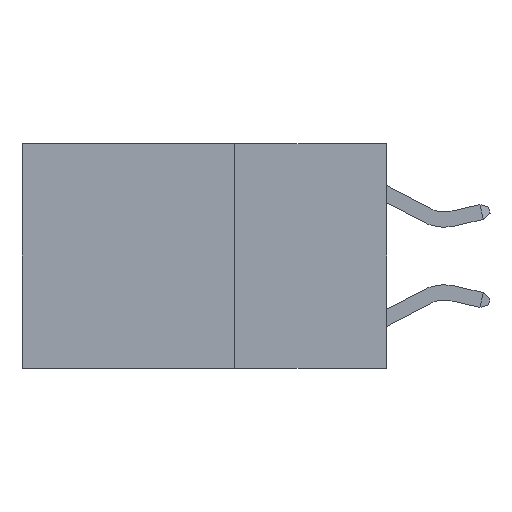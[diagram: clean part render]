
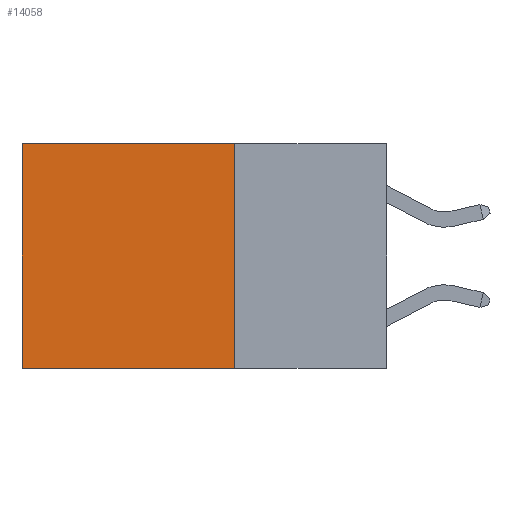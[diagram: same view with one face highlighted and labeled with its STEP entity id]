
A CAD part, left-side view. The second image highlights one B-rep face of the part: STEP entity #14058.
In plain terms, the highlighted planar face has unit normal (-1, 0, 0).
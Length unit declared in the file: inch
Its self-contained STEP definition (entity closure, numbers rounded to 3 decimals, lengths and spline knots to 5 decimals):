
#892 = EDGE_CURVE ( 'NONE', #7675, #2866, #4655, .T. ) ;
#1276 = AXIS2_PLACEMENT_3D ( 'NONE', #11040, #17095, #6116 ) ;
#1988 = EDGE_CURVE ( 'NONE', #10355, #12575, #14997, .T. ) ;
#2866 = VERTEX_POINT ( 'NONE', #5969 ) ;
#3152 = CARTESIAN_POINT ( 'NONE',  ( 0.2625, 0.25, -0.37 ) ) ;
#3820 = VECTOR ( 'NONE', #10582, 39.37008 ) ;
#3821 = EDGE_LOOP ( 'NONE', ( #10452, #7895, #17767, #5028 ) ) ;
#4655 = LINE ( 'NONE', #11535, #8681 ) ;
#4749 = VECTOR ( 'NONE', #5921, 39.37008 ) ;
#5028 = ORIENTED_EDGE ( 'NONE', *, *, #13961, .T. ) ;
#5495 = PLANE ( 'NONE',  #1276 ) ;
#5890 = DIRECTION ( 'NONE',  ( 0., 0., -1. ) ) ;
#5921 = DIRECTION ( 'NONE',  ( 0., 1., 0. ) ) ;
#5969 = CARTESIAN_POINT ( 'NONE',  ( 0.2625, 0.25, -0.37 ) ) ;
#6116 = DIRECTION ( 'NONE',  ( 0., 0., -1. ) ) ;
#6934 = DIRECTION ( 'NONE',  ( 0., 1., 0. ) ) ;
#7675 = VERTEX_POINT ( 'NONE', #14507 ) ;
#7895 = ORIENTED_EDGE ( 'NONE', *, *, #13268, .F. ) ;
#7910 = VECTOR ( 'NONE', #6934, 39.37008 ) ;
#8681 = VECTOR ( 'NONE', #5890, 39.37008 ) ;
#10355 = VERTEX_POINT ( 'NONE', #13495 ) ;
#10452 = ORIENTED_EDGE ( 'NONE', *, *, #1988, .T. ) ;
#10582 = DIRECTION ( 'NONE',  ( 0., 0., -1. ) ) ;
#11040 = CARTESIAN_POINT ( 'NONE',  ( 0.2625, 0.25, 0. ) ) ;
#11535 = CARTESIAN_POINT ( 'NONE',  ( 0.2625, 0.25, 0. ) ) ;
#11789 = CARTESIAN_POINT ( 'NONE',  ( 0.2625, 0.6, 0. ) ) ;
#12575 = VERTEX_POINT ( 'NONE', #15438 ) ;
#13268 = EDGE_CURVE ( 'NONE', #2866, #12575, #15522, .T. ) ;
#13495 = CARTESIAN_POINT ( 'NONE',  ( 0.2625, 0.6, 0. ) ) ;
#13785 = FACE_OUTER_BOUND ( 'NONE', #3821, .T. ) ;
#13961 = EDGE_CURVE ( 'NONE', #7675, #10355, #15163, .T. ) ;
#14058 = ADVANCED_FACE ( 'NONE', ( #13785 ), #5495, .F. ) ;
#14507 = CARTESIAN_POINT ( 'NONE',  ( 0.2625, 0.25, 0. ) ) ;
#14997 = LINE ( 'NONE', #11789, #3820 ) ;
#15163 = LINE ( 'NONE', #15442, #7910 ) ;
#15438 = CARTESIAN_POINT ( 'NONE',  ( 0.2625, 0.6, -0.37 ) ) ;
#15442 = CARTESIAN_POINT ( 'NONE',  ( 0.2625, 0.25, 0. ) ) ;
#15522 = LINE ( 'NONE', #3152, #4749 ) ;
#17095 = DIRECTION ( 'NONE',  ( 1., 0., 0. ) ) ;
#17767 = ORIENTED_EDGE ( 'NONE', *, *, #892, .F. ) ;
